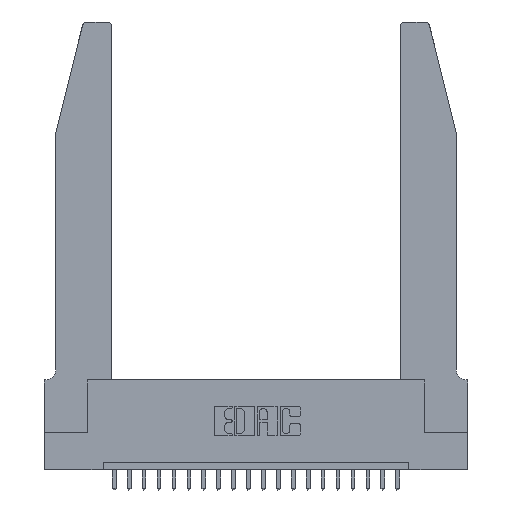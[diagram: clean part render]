
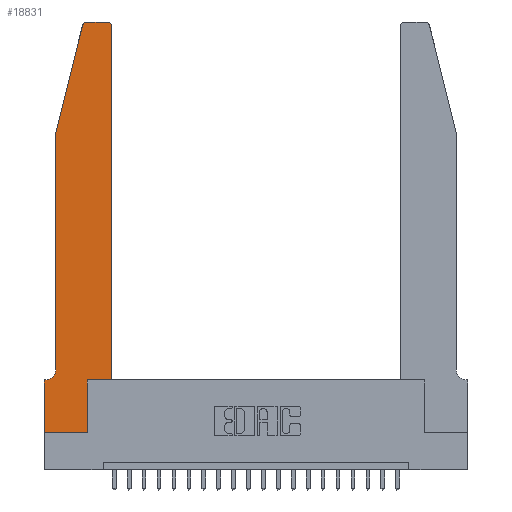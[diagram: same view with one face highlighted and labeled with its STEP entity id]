
A CAD part, top view. The second image highlights one B-rep face of the part: STEP entity #18831.
In plain terms, the highlighted planar face has unit normal (0, 0, 1).
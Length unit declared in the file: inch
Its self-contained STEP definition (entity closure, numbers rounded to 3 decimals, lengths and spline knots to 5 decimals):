
#16 = CIRCLE ( 'NONE', #6732, 0.03 ) ;
#275 = DIRECTION ( 'NONE',  ( 0., 0., 1. ) ) ;
#719 = VECTOR ( 'NONE', #6025, 39.37008 ) ;
#742 = LINE ( 'NONE', #14321, #12346 ) ;
#1212 = EDGE_CURVE ( 'NONE', #11019, #19486, #5459, .T. ) ;
#1770 = EDGE_CURVE ( 'NONE', #9896, #11019, #4318, .T. ) ;
#2536 = VECTOR ( 'NONE', #9339, 39.37008 ) ;
#2847 = CARTESIAN_POINT ( 'NONE',  ( 0.2865, 0.35, 0.37 ) ) ;
#3212 = DIRECTION ( 'NONE',  ( 1., 0., 0. ) ) ;
#3232 = CARTESIAN_POINT ( 'NONE',  ( 0.25487, 2.72718, 0.37 ) ) ;
#3584 = ORIENTED_EDGE ( 'NONE', *, *, #8931, .T. ) ;
#3734 = LINE ( 'NONE', #5199, #9506 ) ;
#3967 = EDGE_CURVE ( 'NONE', #7252, #20586, #8661, .T. ) ;
#4318 = LINE ( 'NONE', #13390, #18585 ) ;
#4897 = VERTEX_POINT ( 'NONE', #10682 ) ;
#5045 = CARTESIAN_POINT ( 'NONE',  ( 0.4505, 2.72, 0.37 ) ) ;
#5199 = CARTESIAN_POINT ( 'NONE',  ( 0.0755, 0.35, 0.37 ) ) ;
#5459 = LINE ( 'NONE', #5807, #719 ) ;
#5512 = CARTESIAN_POINT ( 'NONE',  ( 0.4205, 2.75, 0.37 ) ) ;
#5598 = VECTOR ( 'NONE', #6505, 39.37008 ) ;
#5807 = CARTESIAN_POINT ( 'NONE',  ( 0.0755, 2., 0.37 ) ) ;
#5886 = CARTESIAN_POINT ( 'NONE',  ( 0.284, 2.72, 0.37 ) ) ;
#6025 = DIRECTION ( 'NONE',  ( 0., -1., 0. ) ) ;
#6104 = LINE ( 'NONE', #6458, #20356 ) ;
#6120 = LINE ( 'NONE', #21461, #10262 ) ;
#6458 = CARTESIAN_POINT ( 'NONE',  ( 0.2605, 2.75, 0.37 ) ) ;
#6505 = DIRECTION ( 'NONE',  ( 0., 1., 0. ) ) ;
#6528 = DIRECTION ( 'NONE',  ( 1., 0., 0. ) ) ;
#6535 = CARTESIAN_POINT ( 'NONE',  ( 0.4505, 0.35, 0.37 ) ) ;
#6732 = AXIS2_PLACEMENT_3D ( 'NONE', #12894, #275, #16108 ) ;
#6835 = ORIENTED_EDGE ( 'NONE', *, *, #14314, .T. ) ;
#7026 = EDGE_CURVE ( 'NONE', #14346, #8378, #742, .T. ) ;
#7037 = LINE ( 'NONE', #7588, #2536 ) ;
#7252 = VERTEX_POINT ( 'NONE', #6535 ) ;
#7264 = ORIENTED_EDGE ( 'NONE', *, *, #11951, .T. ) ;
#7588 = CARTESIAN_POINT ( 'NONE',  ( 0.4505, 0.35, 0.37 ) ) ;
#7998 = CARTESIAN_POINT ( 'NONE',  ( 0.4505, 0.35, 0.37 ) ) ;
#8378 = VERTEX_POINT ( 'NONE', #13819 ) ;
#8661 = LINE ( 'NONE', #7998, #17123 ) ;
#8714 = DIRECTION ( 'NONE',  ( 0., 0., 1. ) ) ;
#8931 = EDGE_CURVE ( 'NONE', #16658, #14346, #3734, .T. ) ;
#9339 = DIRECTION ( 'NONE',  ( 1., 0., 0. ) ) ;
#9414 = ORIENTED_EDGE ( 'NONE', *, *, #1212, .T. ) ;
#9506 = VECTOR ( 'NONE', #15619, 39.37008 ) ;
#9896 = VERTEX_POINT ( 'NONE', #3232 ) ;
#10248 = CARTESIAN_POINT ( 'NONE',  ( 0., 0.35, 0.37 ) ) ;
#10262 = VECTOR ( 'NONE', #6528, 39.37008 ) ;
#10403 = PLANE ( 'NONE',  #19145 ) ;
#10545 = EDGE_LOOP ( 'NONE', ( #7264, #11135, #10615, #9414, #22488, #3584, #22229, #18431, #22111, #6835, #10569, #14205 ) ) ;
#10569 = ORIENTED_EDGE ( 'NONE', *, *, #3967, .T. ) ;
#10615 = ORIENTED_EDGE ( 'NONE', *, *, #1770, .T. ) ;
#10682 = CARTESIAN_POINT ( 'NONE',  ( 0.2865, 0.35, 0.37 ) ) ;
#10780 = CARTESIAN_POINT ( 'NONE',  ( 0.2865, 0., 0.37 ) ) ;
#10835 = EDGE_CURVE ( 'NONE', #8378, #21319, #6120, .T. ) ;
#10915 = CARTESIAN_POINT ( 'NONE',  ( 0.0755, 2., 0.37 ) ) ;
#11019 = VERTEX_POINT ( 'NONE', #10915 ) ;
#11135 = ORIENTED_EDGE ( 'NONE', *, *, #15431, .T. ) ;
#11847 = EDGE_CURVE ( 'NONE', #20586, #14216, #16, .T. ) ;
#11951 = EDGE_CURVE ( 'NONE', #14216, #22196, #6104, .T. ) ;
#11994 = EDGE_CURVE ( 'NONE', #19486, #16658, #14336, .T. ) ;
#12200 = AXIS2_PLACEMENT_3D ( 'NONE', #5886, #16663, #18149 ) ;
#12346 = VECTOR ( 'NONE', #17997, 39.37008 ) ;
#12780 = CARTESIAN_POINT ( 'NONE',  ( 0., 0.35, 0.37 ) ) ;
#12894 = CARTESIAN_POINT ( 'NONE',  ( 0.4205, 2.72, 0.37 ) ) ;
#12995 = LINE ( 'NONE', #2847, #5598 ) ;
#13390 = CARTESIAN_POINT ( 'NONE',  ( 0.0755, 2., 0.37 ) ) ;
#13819 = CARTESIAN_POINT ( 'NONE',  ( 0., 0., 0.37 ) ) ;
#13958 = CARTESIAN_POINT ( 'NONE',  ( 0.0755, 0.42, 0.37 ) ) ;
#14205 = ORIENTED_EDGE ( 'NONE', *, *, #11847, .T. ) ;
#14216 = VERTEX_POINT ( 'NONE', #5512 ) ;
#14314 = EDGE_CURVE ( 'NONE', #4897, #7252, #7037, .T. ) ;
#14321 = CARTESIAN_POINT ( 'NONE',  ( 0., 0., 0.37 ) ) ;
#14336 = CIRCLE ( 'NONE', #16966, 0.07 ) ;
#14346 = VERTEX_POINT ( 'NONE', #12780 ) ;
#14358 = CIRCLE ( 'NONE', #12200, 0.03 ) ;
#15023 = DIRECTION ( 'NONE',  ( 0., 1., 0. ) ) ;
#15074 = EDGE_CURVE ( 'NONE', #21319, #4897, #12995, .T. ) ;
#15431 = EDGE_CURVE ( 'NONE', #22196, #9896, #14358, .T. ) ;
#15438 = FACE_OUTER_BOUND ( 'NONE', #10545, .T. ) ;
#15619 = DIRECTION ( 'NONE',  ( -1., 0., 0. ) ) ;
#16108 = DIRECTION ( 'NONE',  ( 1., 0., 0. ) ) ;
#16658 = VERTEX_POINT ( 'NONE', #22736 ) ;
#16663 = DIRECTION ( 'NONE',  ( 0., 0., 1. ) ) ;
#16966 = AXIS2_PLACEMENT_3D ( 'NONE', #20859, #19241, #22566 ) ;
#17123 = VECTOR ( 'NONE', #15023, 39.37008 ) ;
#17997 = DIRECTION ( 'NONE',  ( 0., -1., 0. ) ) ;
#18149 = DIRECTION ( 'NONE',  ( 1., 0., 0. ) ) ;
#18431 = ORIENTED_EDGE ( 'NONE', *, *, #10835, .T. ) ;
#18585 = VECTOR ( 'NONE', #20152, 39.37008 ) ;
#18746 = CARTESIAN_POINT ( 'NONE',  ( 0.284, 2.75, 0.37 ) ) ;
#18831 = ADVANCED_FACE ( 'NONE', ( #15438 ), #10403, .T. ) ;
#19145 = AXIS2_PLACEMENT_3D ( 'NONE', #10248, #8714, #3212 ) ;
#19241 = DIRECTION ( 'NONE',  ( 0., 0., -1. ) ) ;
#19486 = VERTEX_POINT ( 'NONE', #13958 ) ;
#20152 = DIRECTION ( 'NONE',  ( -0.239, -0.971, 0. ) ) ;
#20356 = VECTOR ( 'NONE', #22259, 39.37008 ) ;
#20586 = VERTEX_POINT ( 'NONE', #5045 ) ;
#20859 = CARTESIAN_POINT ( 'NONE',  ( 0.0055, 0.42, 0.37 ) ) ;
#21319 = VERTEX_POINT ( 'NONE', #10780 ) ;
#21461 = CARTESIAN_POINT ( 'NONE',  ( 0., 0., 0.37 ) ) ;
#22111 = ORIENTED_EDGE ( 'NONE', *, *, #15074, .T. ) ;
#22196 = VERTEX_POINT ( 'NONE', #18746 ) ;
#22229 = ORIENTED_EDGE ( 'NONE', *, *, #7026, .T. ) ;
#22259 = DIRECTION ( 'NONE',  ( -1., 0., 0. ) ) ;
#22488 = ORIENTED_EDGE ( 'NONE', *, *, #11994, .T. ) ;
#22566 = DIRECTION ( 'NONE',  ( -1., 0., 0. ) ) ;
#22736 = CARTESIAN_POINT ( 'NONE',  ( 0.0055, 0.35, 0.37 ) ) ;
